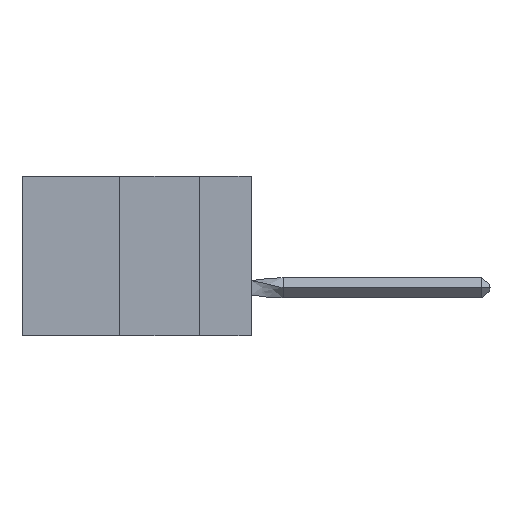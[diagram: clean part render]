
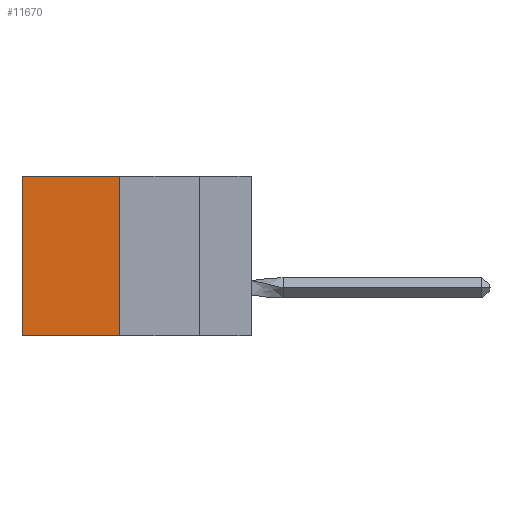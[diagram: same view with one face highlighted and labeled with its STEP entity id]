
A CAD part, left-side view. The second image highlights one B-rep face of the part: STEP entity #11670.
In plain terms, the highlighted planar face has unit normal (-1, 0, 0).
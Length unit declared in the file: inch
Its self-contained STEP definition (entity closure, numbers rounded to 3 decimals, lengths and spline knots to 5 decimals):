
#292 = FACE_OUTER_BOUND ( 'NONE', #8509, .T. ) ;
#1218 = CARTESIAN_POINT ( 'NONE',  ( 0.305, 0.72, 0. ) ) ;
#2240 = VERTEX_POINT ( 'NONE', #10403 ) ;
#2648 = ORIENTED_EDGE ( 'NONE', *, *, #9467, .F. ) ;
#2898 = VECTOR ( 'NONE', #14802, 39.37008 ) ;
#3203 = CARTESIAN_POINT ( 'NONE',  ( 0.305, 0.413, -0.5 ) ) ;
#3606 = VECTOR ( 'NONE', #11484, 39.37008 ) ;
#5087 = CARTESIAN_POINT ( 'NONE',  ( 0.305, 0.72, -0.5 ) ) ;
#5876 = ORIENTED_EDGE ( 'NONE', *, *, #11001, .T. ) ;
#6017 = LINE ( 'NONE', #11377, #2898 ) ;
#6409 = LINE ( 'NONE', #8224, #6605 ) ;
#6439 = CARTESIAN_POINT ( 'NONE',  ( 0.305, 0.413, 0. ) ) ;
#6605 = VECTOR ( 'NONE', #13012, 39.37008 ) ;
#6903 = VERTEX_POINT ( 'NONE', #6439 ) ;
#7605 = VERTEX_POINT ( 'NONE', #10206 ) ;
#7697 = VERTEX_POINT ( 'NONE', #1218 ) ;
#7908 = EDGE_CURVE ( 'NONE', #6903, #7697, #6409, .T. ) ;
#8224 = CARTESIAN_POINT ( 'NONE',  ( 0.305, 0.413, 0. ) ) ;
#8509 = EDGE_LOOP ( 'NONE', ( #5876, #2648, #13078, #14545 ) ) ;
#8702 = DIRECTION ( 'NONE',  ( 0., 0., -1. ) ) ;
#8898 = DIRECTION ( 'NONE',  ( 1., 0., 0. ) ) ;
#8999 = PLANE ( 'NONE',  #11675 ) ;
#9215 = VECTOR ( 'NONE', #8702, 39.37008 ) ;
#9364 = EDGE_CURVE ( 'NONE', #6903, #7605, #6017, .T. ) ;
#9467 = EDGE_CURVE ( 'NONE', #7605, #2240, #13429, .T. ) ;
#10206 = CARTESIAN_POINT ( 'NONE',  ( 0.305, 0.413, -0.5 ) ) ;
#10403 = CARTESIAN_POINT ( 'NONE',  ( 0.305, 0.72, -0.5 ) ) ;
#11001 = EDGE_CURVE ( 'NONE', #7697, #2240, #14667, .T. ) ;
#11377 = CARTESIAN_POINT ( 'NONE',  ( 0.305, 0.413, -0.5 ) ) ;
#11484 = DIRECTION ( 'NONE',  ( 0., 1., 0. ) ) ;
#11670 = ADVANCED_FACE ( 'NONE', ( #292 ), #8999, .F. ) ;
#11675 = AXIS2_PLACEMENT_3D ( 'NONE', #3203, #8898, #12545 ) ;
#12545 = DIRECTION ( 'NONE',  ( 0., 0., -1. ) ) ;
#13012 = DIRECTION ( 'NONE',  ( 0., 1., 0. ) ) ;
#13078 = ORIENTED_EDGE ( 'NONE', *, *, #9364, .F. ) ;
#13429 = LINE ( 'NONE', #14966, #3606 ) ;
#14545 = ORIENTED_EDGE ( 'NONE', *, *, #7908, .T. ) ;
#14667 = LINE ( 'NONE', #5087, #9215 ) ;
#14802 = DIRECTION ( 'NONE',  ( 0., 0., -1. ) ) ;
#14966 = CARTESIAN_POINT ( 'NONE',  ( 0.305, 0.413, -0.5 ) ) ;
